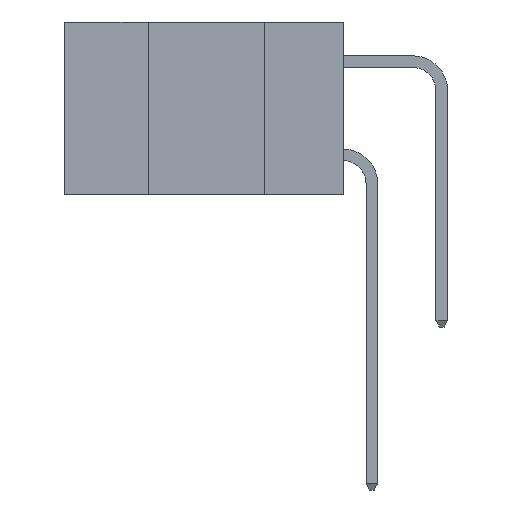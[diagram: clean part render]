
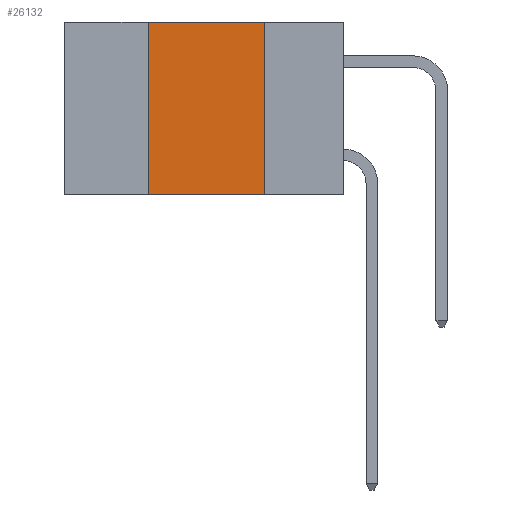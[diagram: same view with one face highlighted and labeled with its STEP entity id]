
A CAD part, left-side view. The second image highlights one B-rep face of the part: STEP entity #26132.
In plain terms, the highlighted planar face has unit normal (-1, 0, 0).
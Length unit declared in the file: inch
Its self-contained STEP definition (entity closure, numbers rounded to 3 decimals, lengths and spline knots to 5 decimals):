
#237 = ORIENTED_EDGE ( 'NONE', *, *, #24903, .F. ) ;
#512 = LINE ( 'NONE', #24882, #1894 ) ;
#1894 = VECTOR ( 'NONE', #24824, 39.37008 ) ;
#2357 = CARTESIAN_POINT ( 'NONE',  ( 0., 0.6, 0. ) ) ;
#3027 = EDGE_CURVE ( 'NONE', #5878, #17842, #512, .T. ) ;
#4537 = DIRECTION ( 'NONE',  ( 0., 0., -1. ) ) ;
#5878 = VERTEX_POINT ( 'NONE', #15264 ) ;
#6427 = VERTEX_POINT ( 'NONE', #18907 ) ;
#6552 = PLANE ( 'NONE',  #25765 ) ;
#7390 = ORIENTED_EDGE ( 'NONE', *, *, #15130, .F. ) ;
#8935 = FACE_OUTER_BOUND ( 'NONE', #14224, .T. ) ;
#9395 = EDGE_CURVE ( 'NONE', #14341, #17842, #19251, .T. ) ;
#10346 = CARTESIAN_POINT ( 'NONE',  ( 0., 0.17, -0.37 ) ) ;
#13586 = CARTESIAN_POINT ( 'NONE',  ( 0., 0.6, 0. ) ) ;
#14074 = VECTOR ( 'NONE', #19886, 39.37008 ) ;
#14224 = EDGE_LOOP ( 'NONE', ( #24570, #237, #7390, #24893 ) ) ;
#14341 = VERTEX_POINT ( 'NONE', #26530 ) ;
#14515 = CARTESIAN_POINT ( 'NONE',  ( 0., 0.42, -0.37 ) ) ;
#15130 = EDGE_CURVE ( 'NONE', #14341, #6427, #26791, .T. ) ;
#15264 = CARTESIAN_POINT ( 'NONE',  ( 0., 0.17, 0. ) ) ;
#15778 = CARTESIAN_POINT ( 'NONE',  ( 0., 0.6, -0.37 ) ) ;
#15784 = VECTOR ( 'NONE', #26920, 39.37008 ) ;
#17371 = DIRECTION ( 'NONE',  ( 1., 0., 0. ) ) ;
#17842 = VERTEX_POINT ( 'NONE', #10346 ) ;
#18907 = CARTESIAN_POINT ( 'NONE',  ( 0., 0.42, 0. ) ) ;
#19251 = LINE ( 'NONE', #15778, #20580 ) ;
#19617 = LINE ( 'NONE', #13586, #14074 ) ;
#19858 = DIRECTION ( 'NONE',  ( 0., -1., 0. ) ) ;
#19886 = DIRECTION ( 'NONE',  ( 0., -1., 0. ) ) ;
#20580 = VECTOR ( 'NONE', #19858, 39.37008 ) ;
#24570 = ORIENTED_EDGE ( 'NONE', *, *, #3027, .F. ) ;
#24824 = DIRECTION ( 'NONE',  ( 0., 0., -1. ) ) ;
#24882 = CARTESIAN_POINT ( 'NONE',  ( 0., 0.17, -0.37 ) ) ;
#24893 = ORIENTED_EDGE ( 'NONE', *, *, #9395, .T. ) ;
#24903 = EDGE_CURVE ( 'NONE', #6427, #5878, #19617, .T. ) ;
#25765 = AXIS2_PLACEMENT_3D ( 'NONE', #2357, #17371, #4537 ) ;
#26132 = ADVANCED_FACE ( 'NONE', ( #8935 ), #6552, .F. ) ;
#26530 = CARTESIAN_POINT ( 'NONE',  ( 0., 0.42, -0.37 ) ) ;
#26791 = LINE ( 'NONE', #14515, #15784 ) ;
#26920 = DIRECTION ( 'NONE',  ( 0., 0., 1. ) ) ;
